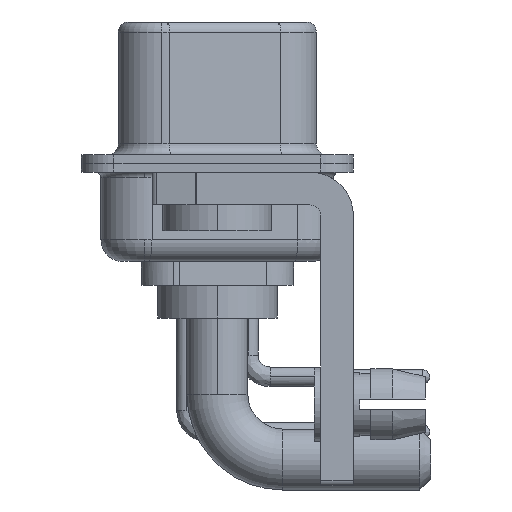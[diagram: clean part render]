
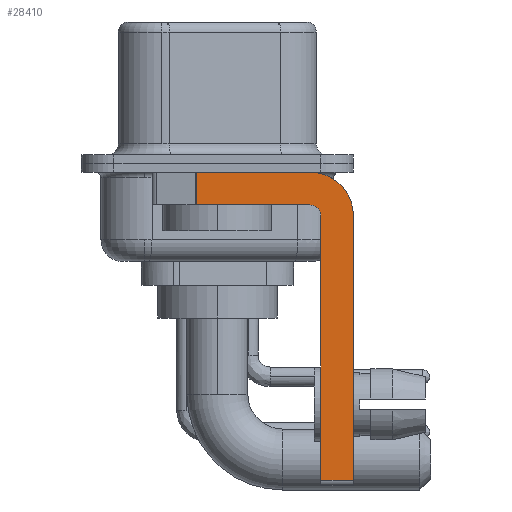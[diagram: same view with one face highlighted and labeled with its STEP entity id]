
A CAD part, left-side view. The second image highlights one B-rep face of the part: STEP entity #28410.
In plain terms, the highlighted planar face has unit normal (-1, 0, 0).
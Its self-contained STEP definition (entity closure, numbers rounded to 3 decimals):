
#377 = AXIS2_PLACEMENT_3D ( 'NONE', #18450, #16450, #13991 ) ;
#887 = CARTESIAN_POINT ( 'NONE',  ( -2.9, 0.978, -1.9 ) ) ;
#1461 = CARTESIAN_POINT ( 'NONE',  ( -2.9, -4.75, -2.4 ) ) ;
#1623 = PLANE ( 'NONE',  #3832 ) ;
#2238 = DIRECTION ( 'NONE',  ( 0., 0., -1. ) ) ;
#2715 = CARTESIAN_POINT ( 'NONE',  ( -2.9, 3., -0.4 ) ) ;
#2741 = VERTEX_POINT ( 'NONE', #13075 ) ;
#2965 = EDGE_LOOP ( 'NONE', ( #25263, #25194, #15060, #7790, #23358, #14088, #28669, #7054 ) ) ;
#3585 = VERTEX_POINT ( 'NONE', #12407 ) ;
#3832 = AXIS2_PLACEMENT_3D ( 'NONE', #6569, #4554, #2238 ) ;
#4374 = VERTEX_POINT ( 'NONE', #27926 ) ;
#4554 = DIRECTION ( 'NONE',  ( 1., 0., 0. ) ) ;
#4885 = AXIS2_PLACEMENT_3D ( 'NONE', #8974, #18487, #8667 ) ;
#5554 = DIRECTION ( 'NONE',  ( 0., 1., 0. ) ) ;
#6352 = EDGE_CURVE ( 'NONE', #27921, #17312, #7245, .T. ) ;
#6375 = LINE ( 'NONE', #18519, #23665 ) ;
#6569 = CARTESIAN_POINT ( 'NONE',  ( -2.9, -4.25, -2.4 ) ) ;
#6799 = VECTOR ( 'NONE', #28668, 1000. ) ;
#6857 = CARTESIAN_POINT ( 'NONE',  ( -2.9, 0.978, -0.4 ) ) ;
#7054 = ORIENTED_EDGE ( 'NONE', *, *, #27891, .F. ) ;
#7088 = CARTESIAN_POINT ( 'NONE',  ( -2.9, -4.75, -14.8 ) ) ;
#7245 = LINE ( 'NONE', #28518, #15383 ) ;
#7686 = LINE ( 'NONE', #7088, #12792 ) ;
#7790 = ORIENTED_EDGE ( 'NONE', *, *, #30474, .F. ) ;
#8012 = LINE ( 'NONE', #887, #6799 ) ;
#8286 = CIRCLE ( 'NONE', #377, 2. ) ;
#8667 = DIRECTION ( 'NONE',  ( 0., 0., 1. ) ) ;
#8974 = CARTESIAN_POINT ( 'NONE',  ( -2.9, -4.25, -2.4 ) ) ;
#9326 = LINE ( 'NONE', #9630, #15754 ) ;
#9630 = CARTESIAN_POINT ( 'NONE',  ( -2.9, -4.25, -14.55 ) ) ;
#9804 = LINE ( 'NONE', #2715, #22147 ) ;
#11258 = EDGE_CURVE ( 'NONE', #24074, #4374, #9326, .T. ) ;
#11529 = DIRECTION ( 'NONE',  ( 0., -1., 0. ) ) ;
#12407 = CARTESIAN_POINT ( 'NONE',  ( -2.9, -6.25, -2.4 ) ) ;
#12792 = VECTOR ( 'NONE', #17065, 1000. ) ;
#13075 = CARTESIAN_POINT ( 'NONE',  ( -2.9, -4.25, -0.4 ) ) ;
#13991 = DIRECTION ( 'NONE',  ( 0., 0., -1. ) ) ;
#14088 = ORIENTED_EDGE ( 'NONE', *, *, #11258, .T. ) ;
#15060 = ORIENTED_EDGE ( 'NONE', *, *, #6352, .F. ) ;
#15383 = VECTOR ( 'NONE', #5554, 1000. ) ;
#15754 = VECTOR ( 'NONE', #16546, 1000. ) ;
#16450 = DIRECTION ( 'NONE',  ( 1., 0., 0. ) ) ;
#16546 = DIRECTION ( 'NONE',  ( 0., -1., 0. ) ) ;
#17065 = DIRECTION ( 'NONE',  ( 0., 0., 1. ) ) ;
#17183 = EDGE_CURVE ( 'NONE', #3585, #4374, #6375, .T. ) ;
#17312 = VERTEX_POINT ( 'NONE', #21153 ) ;
#17847 = CARTESIAN_POINT ( 'NONE',  ( -2.9, -4.75, -14.55 ) ) ;
#18450 = CARTESIAN_POINT ( 'NONE',  ( -2.9, -4.25, -2.4 ) ) ;
#18487 = DIRECTION ( 'NONE',  ( -1., 0., 0. ) ) ;
#18519 = CARTESIAN_POINT ( 'NONE',  ( -2.9, -6.25, -2.4 ) ) ;
#20785 = CARTESIAN_POINT ( 'NONE',  ( -2.9, -4.25, -1.9 ) ) ;
#21153 = CARTESIAN_POINT ( 'NONE',  ( -2.9, 0.978, -1.9 ) ) ;
#22147 = VECTOR ( 'NONE', #11529, 1000. ) ;
#22600 = CIRCLE ( 'NONE', #4885, 0.5 ) ;
#22876 = DIRECTION ( 'NONE',  ( 0., 0., -1. ) ) ;
#23358 = ORIENTED_EDGE ( 'NONE', *, *, #25971, .F. ) ;
#23665 = VECTOR ( 'NONE', #22876, 1000. ) ;
#24074 = VERTEX_POINT ( 'NONE', #17847 ) ;
#24249 = EDGE_CURVE ( 'NONE', #28409, #2741, #9804, .T. ) ;
#25194 = ORIENTED_EDGE ( 'NONE', *, *, #27726, .T. ) ;
#25263 = ORIENTED_EDGE ( 'NONE', *, *, #24249, .F. ) ;
#25685 = FACE_OUTER_BOUND ( 'NONE', #2965, .T. ) ;
#25971 = EDGE_CURVE ( 'NONE', #24074, #28280, #7686, .T. ) ;
#27726 = EDGE_CURVE ( 'NONE', #28409, #17312, #8012, .T. ) ;
#27891 = EDGE_CURVE ( 'NONE', #2741, #3585, #8286, .T. ) ;
#27921 = VERTEX_POINT ( 'NONE', #20785 ) ;
#27926 = CARTESIAN_POINT ( 'NONE',  ( -2.9, -6.25, -14.55 ) ) ;
#28280 = VERTEX_POINT ( 'NONE', #1461 ) ;
#28409 = VERTEX_POINT ( 'NONE', #6857 ) ;
#28410 = ADVANCED_FACE ( 'NONE', ( #25685 ), #1623, .F. ) ;
#28518 = CARTESIAN_POINT ( 'NONE',  ( -2.9, -4.25, -1.9 ) ) ;
#28668 = DIRECTION ( 'NONE',  ( 0., 0., -1. ) ) ;
#28669 = ORIENTED_EDGE ( 'NONE', *, *, #17183, .F. ) ;
#30474 = EDGE_CURVE ( 'NONE', #28280, #27921, #22600, .T. ) ;
